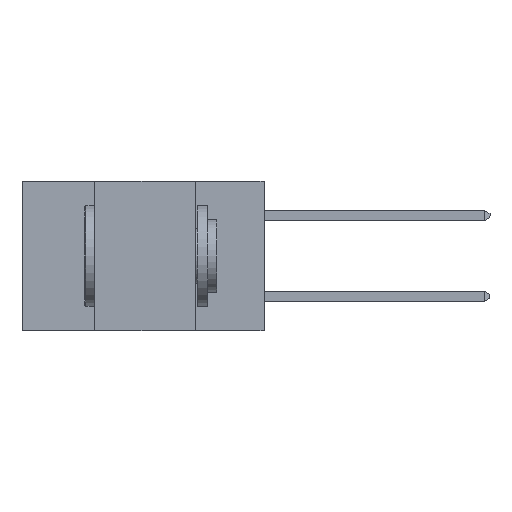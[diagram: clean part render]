
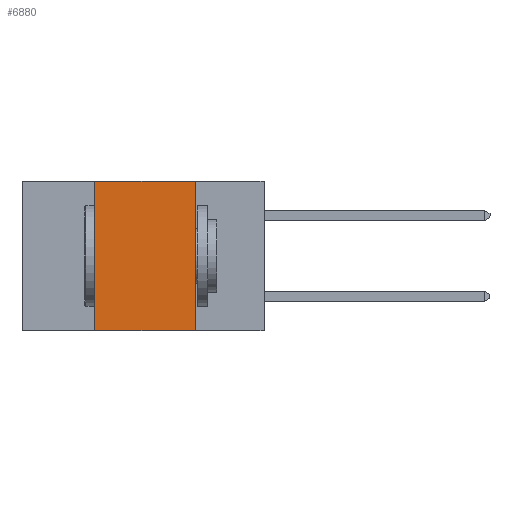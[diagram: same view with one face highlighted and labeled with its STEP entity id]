
A CAD part, left-side view. The second image highlights one B-rep face of the part: STEP entity #6880.
In plain terms, the highlighted planar face has unit normal (-1, 0, 0).
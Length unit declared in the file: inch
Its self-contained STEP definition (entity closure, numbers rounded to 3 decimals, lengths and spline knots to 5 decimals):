
#380 = EDGE_CURVE ( 'NONE', #5342, #25011, #11018, .T. ) ;
#2850 = CARTESIAN_POINT ( 'NONE',  ( 0., 0.6, 0. ) ) ;
#3294 = CARTESIAN_POINT ( 'NONE',  ( 0., 0.17, 0. ) ) ;
#3394 = CARTESIAN_POINT ( 'NONE',  ( 0., 0.42, -0.37 ) ) ;
#4376 = VECTOR ( 'NONE', #15913, 39.37008 ) ;
#4464 = VERTEX_POINT ( 'NONE', #3394 ) ;
#5342 = VERTEX_POINT ( 'NONE', #22054 ) ;
#5535 = CARTESIAN_POINT ( 'NONE',  ( 0., 0.42, 0. ) ) ;
#6880 = ADVANCED_FACE ( 'NONE', ( #9022 ), #13062, .F. ) ;
#8138 = VECTOR ( 'NONE', #11068, 39.37008 ) ;
#8615 = CARTESIAN_POINT ( 'NONE',  ( 0., 0.42, 0. ) ) ;
#8922 = CARTESIAN_POINT ( 'NONE',  ( 0., 0.6, -0.37 ) ) ;
#9022 = FACE_OUTER_BOUND ( 'NONE', #19808, .T. ) ;
#11018 = LINE ( 'NONE', #3294, #4376 ) ;
#11068 = DIRECTION ( 'NONE',  ( 0., -1., 0. ) ) ;
#11193 = CARTESIAN_POINT ( 'NONE',  ( 0., 0.17, -0.37 ) ) ;
#11957 = EDGE_CURVE ( 'NONE', #4464, #25189, #18754, .T. ) ;
#13062 = PLANE ( 'NONE',  #20948 ) ;
#13217 = DIRECTION ( 'NONE',  ( 1., 0., 0. ) ) ;
#13257 = CARTESIAN_POINT ( 'NONE',  ( 0., 0.6, 0. ) ) ;
#13633 = DIRECTION ( 'NONE',  ( 0., 0., -1. ) ) ;
#15913 = DIRECTION ( 'NONE',  ( 0., 0., -1. ) ) ;
#15953 = ORIENTED_EDGE ( 'NONE', *, *, #380, .F. ) ;
#16067 = ORIENTED_EDGE ( 'NONE', *, *, #21274, .F. ) ;
#16364 = ORIENTED_EDGE ( 'NONE', *, *, #11957, .F. ) ;
#16432 = ORIENTED_EDGE ( 'NONE', *, *, #16921, .T. ) ;
#16921 = EDGE_CURVE ( 'NONE', #4464, #25011, #19961, .T. ) ;
#18420 = DIRECTION ( 'NONE',  ( 0., -1., 0. ) ) ;
#18754 = LINE ( 'NONE', #8615, #26089 ) ;
#19808 = EDGE_LOOP ( 'NONE', ( #15953, #16067, #16364, #16432 ) ) ;
#19961 = LINE ( 'NONE', #8922, #8138 ) ;
#20948 = AXIS2_PLACEMENT_3D ( 'NONE', #13257, #13217, #13633 ) ;
#21274 = EDGE_CURVE ( 'NONE', #25189, #5342, #27254, .T. ) ;
#22054 = CARTESIAN_POINT ( 'NONE',  ( 0., 0.17, 0. ) ) ;
#22743 = VECTOR ( 'NONE', #18420, 39.37008 ) ;
#24183 = DIRECTION ( 'NONE',  ( 0., 0., 1. ) ) ;
#25011 = VERTEX_POINT ( 'NONE', #11193 ) ;
#25189 = VERTEX_POINT ( 'NONE', #5535 ) ;
#26089 = VECTOR ( 'NONE', #24183, 39.37008 ) ;
#27254 = LINE ( 'NONE', #2850, #22743 ) ;
